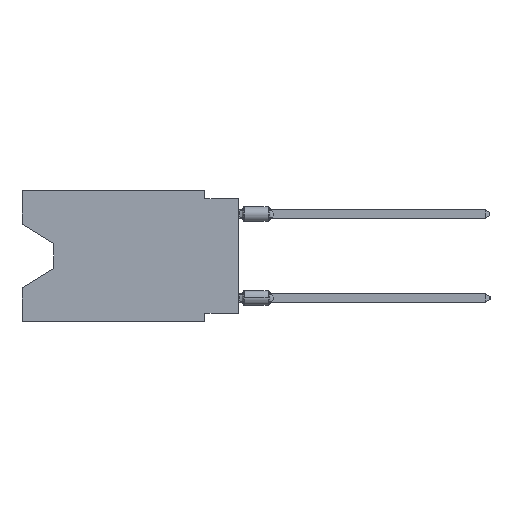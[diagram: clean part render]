
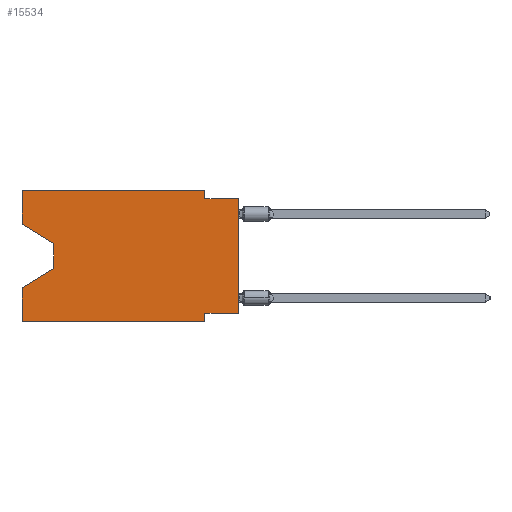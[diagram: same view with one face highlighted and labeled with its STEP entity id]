
A CAD part, left-side view. The second image highlights one B-rep face of the part: STEP entity #15534.
In plain terms, the highlighted planar face has unit normal (-1, 0, 0).
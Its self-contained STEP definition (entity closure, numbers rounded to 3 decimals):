
#346 = LINE ( 'NONE', #48675, #11866 ) ;
#2609 = ORIENTED_EDGE ( 'NONE', *, *, #58364, .T. ) ;
#3187 = VERTEX_POINT ( 'NONE', #8969 ) ;
#3263 = DIRECTION ( 'NONE',  ( 0., 0., -1. ) ) ;
#3707 = VERTEX_POINT ( 'NONE', #16594 ) ;
#4147 = EDGE_CURVE ( 'NONE', #46328, #3187, #7429, .T. ) ;
#4243 = EDGE_CURVE ( 'NONE', #21112, #31485, #32195, .T. ) ;
#4517 = CARTESIAN_POINT ( 'NONE',  ( 0., 16.383, -9.906 ) ) ;
#4844 = DIRECTION ( 'NONE',  ( 1., 0., 0. ) ) ;
#5967 = DIRECTION ( 'NONE',  ( 0., -1., 0. ) ) ;
#6105 = VECTOR ( 'NONE', #41032, 1000. ) ;
#6483 = VECTOR ( 'NONE', #56384, 1000. ) ;
#6961 = CARTESIAN_POINT ( 'NONE',  ( 0., 16.383, -2.546 ) ) ;
#7369 = ORIENTED_EDGE ( 'NONE', *, *, #18005, .T. ) ;
#7429 = LINE ( 'NONE', #17142, #6105 ) ;
#7562 = CARTESIAN_POINT ( 'NONE',  ( 0., 2.54, -9.906 ) ) ;
#8344 = CARTESIAN_POINT ( 'NONE',  ( 0., 2.54, 0. ) ) ;
#8715 = EDGE_CURVE ( 'NONE', #44146, #16045, #46496, .T. ) ;
#8969 = CARTESIAN_POINT ( 'NONE',  ( 0., 16.383, 0. ) ) ;
#9037 = VERTEX_POINT ( 'NONE', #61860 ) ;
#9397 = AXIS2_PLACEMENT_3D ( 'NONE', #21029, #4844, #15163 ) ;
#9402 = EDGE_LOOP ( 'NONE', ( #2609, #38837, #22296, #36250, #7369, #38376, #29095, #37198, #37294, #35481, #54092, #39087 ) ) ;
#9856 = PLANE ( 'NONE',  #9397 ) ;
#10104 = VERTEX_POINT ( 'NONE', #50363 ) ;
#11655 = DIRECTION ( 'NONE',  ( 0., -0.855, -0.519 ) ) ;
#11844 = CARTESIAN_POINT ( 'NONE',  ( 0., 0., -9.271 ) ) ;
#11866 = VECTOR ( 'NONE', #5967, 1000. ) ;
#13773 = VECTOR ( 'NONE', #52281, 1000. ) ;
#13966 = CARTESIAN_POINT ( 'NONE',  ( 0., 16.383, -9.906 ) ) ;
#15163 = DIRECTION ( 'NONE',  ( 0., 0., -1. ) ) ;
#15534 = ADVANCED_FACE ( 'NONE', ( #34003 ), #9856, .F. ) ;
#16045 = VERTEX_POINT ( 'NONE', #45458 ) ;
#16594 = CARTESIAN_POINT ( 'NONE',  ( 0., 2.54, 0. ) ) ;
#16851 = EDGE_CURVE ( 'NONE', #41523, #10104, #21306, .T. ) ;
#17142 = CARTESIAN_POINT ( 'NONE',  ( 0., 16.383, 0. ) ) ;
#17766 = DIRECTION ( 'NONE',  ( 0., 0., 1. ) ) ;
#18005 = EDGE_CURVE ( 'NONE', #41523, #16045, #47525, .T. ) ;
#19698 = CARTESIAN_POINT ( 'NONE',  ( 0., 0., -9.271 ) ) ;
#20582 = VECTOR ( 'NONE', #11655, 1000. ) ;
#21029 = CARTESIAN_POINT ( 'NONE',  ( 0., 16.383, 0. ) ) ;
#21112 = VERTEX_POINT ( 'NONE', #11844 ) ;
#21306 = LINE ( 'NONE', #35761, #37399 ) ;
#22296 = ORIENTED_EDGE ( 'NONE', *, *, #61144, .T. ) ;
#23993 = LINE ( 'NONE', #8344, #6483 ) ;
#24644 = DIRECTION ( 'NONE',  ( 0., -1., 0. ) ) ;
#25654 = EDGE_CURVE ( 'NONE', #48713, #31485, #48543, .T. ) ;
#29052 = EDGE_CURVE ( 'NONE', #61599, #9037, #40943, .T. ) ;
#29095 = ORIENTED_EDGE ( 'NONE', *, *, #44173, .F. ) ;
#31485 = VERTEX_POINT ( 'NONE', #43900 ) ;
#32195 = LINE ( 'NONE', #51390, #51246 ) ;
#34003 = FACE_OUTER_BOUND ( 'NONE', #9402, .T. ) ;
#34313 = VECTOR ( 'NONE', #47687, 1000. ) ;
#35161 = VECTOR ( 'NONE', #24644, 1000. ) ;
#35463 = VECTOR ( 'NONE', #42813, 1000. ) ;
#35481 = ORIENTED_EDGE ( 'NONE', *, *, #48664, .F. ) ;
#35761 = CARTESIAN_POINT ( 'NONE',  ( 0., 16.383, 0. ) ) ;
#36125 = DIRECTION ( 'NONE',  ( 0., 0., -1. ) ) ;
#36250 = ORIENTED_EDGE ( 'NONE', *, *, #16851, .F. ) ;
#37138 = CARTESIAN_POINT ( 'NONE',  ( 0., 13.97, -4.013 ) ) ;
#37198 = ORIENTED_EDGE ( 'NONE', *, *, #4243, .T. ) ;
#37294 = ORIENTED_EDGE ( 'NONE', *, *, #25654, .F. ) ;
#37399 = VECTOR ( 'NONE', #59643, 1000. ) ;
#38376 = ORIENTED_EDGE ( 'NONE', *, *, #8715, .F. ) ;
#38837 = ORIENTED_EDGE ( 'NONE', *, *, #29052, .T. ) ;
#39087 = ORIENTED_EDGE ( 'NONE', *, *, #4147, .F. ) ;
#40943 = LINE ( 'NONE', #37138, #60264 ) ;
#41032 = DIRECTION ( 'NONE',  ( 0., 0., 1. ) ) ;
#41523 = VERTEX_POINT ( 'NONE', #13966 ) ;
#41946 = CARTESIAN_POINT ( 'NONE',  ( 0., 2.54, -0.635 ) ) ;
#42052 = CARTESIAN_POINT ( 'NONE',  ( 0., 2.54, -9.271 ) ) ;
#42563 = VECTOR ( 'NONE', #36125, 1000. ) ;
#42813 = DIRECTION ( 'NONE',  ( 0., -1., 0. ) ) ;
#43900 = CARTESIAN_POINT ( 'NONE',  ( 0., 0., -0.635 ) ) ;
#44146 = VERTEX_POINT ( 'NONE', #42052 ) ;
#44173 = EDGE_CURVE ( 'NONE', #21112, #44146, #51165, .T. ) ;
#45458 = CARTESIAN_POINT ( 'NONE',  ( 0., 2.54, -9.906 ) ) ;
#46328 = VERTEX_POINT ( 'NONE', #6961 ) ;
#46496 = LINE ( 'NONE', #7562, #42563 ) ;
#47296 = CARTESIAN_POINT ( 'NONE',  ( 0., 0., -0.635 ) ) ;
#47525 = LINE ( 'NONE', #4517, #35463 ) ;
#47687 = DIRECTION ( 'NONE',  ( 0., 1., 0. ) ) ;
#48543 = LINE ( 'NONE', #47296, #35161 ) ;
#48664 = EDGE_CURVE ( 'NONE', #3707, #48713, #23993, .T. ) ;
#48675 = CARTESIAN_POINT ( 'NONE',  ( 0., 16.383, 0. ) ) ;
#48713 = VERTEX_POINT ( 'NONE', #41946 ) ;
#50113 = LINE ( 'NONE', #51363, #13773 ) ;
#50363 = CARTESIAN_POINT ( 'NONE',  ( 0., 16.383, -7.36 ) ) ;
#51165 = LINE ( 'NONE', #19698, #34313 ) ;
#51246 = VECTOR ( 'NONE', #17766, 1000. ) ;
#51363 = CARTESIAN_POINT ( 'NONE',  ( 0., 13.97, -5.893 ) ) ;
#51390 = CARTESIAN_POINT ( 'NONE',  ( 0., 0., 0. ) ) ;
#52281 = DIRECTION ( 'NONE',  ( 0., 0.855, -0.519 ) ) ;
#54092 = ORIENTED_EDGE ( 'NONE', *, *, #54096, .F. ) ;
#54096 = EDGE_CURVE ( 'NONE', #3187, #3707, #346, .T. ) ;
#55316 = CARTESIAN_POINT ( 'NONE',  ( 0., 16.383, -2.546 ) ) ;
#56384 = DIRECTION ( 'NONE',  ( 0., 0., -1. ) ) ;
#56536 = CARTESIAN_POINT ( 'NONE',  ( 0., 13.97, -4.013 ) ) ;
#58364 = EDGE_CURVE ( 'NONE', #46328, #61599, #59710, .T. ) ;
#59643 = DIRECTION ( 'NONE',  ( 0., 0., 1. ) ) ;
#59710 = LINE ( 'NONE', #55316, #20582 ) ;
#60264 = VECTOR ( 'NONE', #3263, 1000. ) ;
#61144 = EDGE_CURVE ( 'NONE', #9037, #10104, #50113, .T. ) ;
#61599 = VERTEX_POINT ( 'NONE', #56536 ) ;
#61860 = CARTESIAN_POINT ( 'NONE',  ( 0., 13.97, -5.893 ) ) ;
